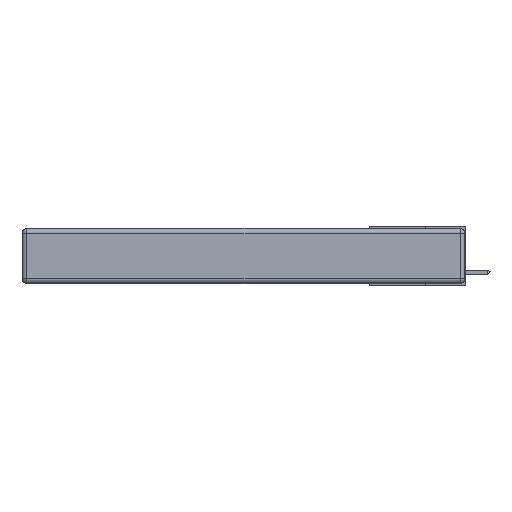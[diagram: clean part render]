
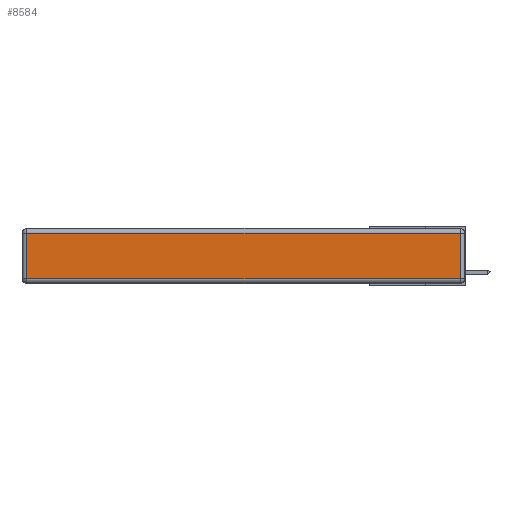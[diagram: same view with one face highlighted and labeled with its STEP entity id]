
A CAD part, left-side view. The second image highlights one B-rep face of the part: STEP entity #8584.
In plain terms, the highlighted planar face has unit normal (-1, 0, 0).
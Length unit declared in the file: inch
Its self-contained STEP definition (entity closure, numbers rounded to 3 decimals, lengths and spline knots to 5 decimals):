
#1359 = EDGE_CURVE ( 'NONE', #32406, #8533, #15320, .T. ) ;
#1415 = EDGE_CURVE ( 'NONE', #8533, #17608, #6360, .T. ) ;
#1460 = LINE ( 'NONE', #2531, #31014 ) ;
#2531 = CARTESIAN_POINT ( 'NONE',  ( 0., 2.75, -0.03 ) ) ;
#3974 = FACE_OUTER_BOUND ( 'NONE', #21183, .T. ) ;
#4182 = DIRECTION ( 'NONE',  ( 0., 0., 1. ) ) ;
#4465 = CARTESIAN_POINT ( 'NONE',  ( 0., 0.03, -0.03 ) ) ;
#6360 = LINE ( 'NONE', #19759, #19071 ) ;
#6834 = DIRECTION ( 'NONE',  ( -1., 0., 0. ) ) ;
#7842 = ORIENTED_EDGE ( 'NONE', *, *, #17301, .T. ) ;
#8352 = VECTOR ( 'NONE', #11616, 39.37008 ) ;
#8439 = ORIENTED_EDGE ( 'NONE', *, *, #1359, .T. ) ;
#8533 = VERTEX_POINT ( 'NONE', #32713 ) ;
#8584 = ADVANCED_FACE ( 'NONE', ( #3974 ), #14493, .T. ) ;
#11616 = DIRECTION ( 'NONE',  ( 0., -1., 0. ) ) ;
#12183 = LINE ( 'NONE', #15162, #33918 ) ;
#13043 = ORIENTED_EDGE ( 'NONE', *, *, #1415, .T. ) ;
#14493 = PLANE ( 'NONE',  #16801 ) ;
#15162 = CARTESIAN_POINT ( 'NONE',  ( 0., 2.72, -0.343 ) ) ;
#15320 = LINE ( 'NONE', #27313, #8352 ) ;
#16801 = AXIS2_PLACEMENT_3D ( 'NONE', #32820, #6834, #4182 ) ;
#17169 = CARTESIAN_POINT ( 'NONE',  ( 0., 2.72, -0.03 ) ) ;
#17209 = EDGE_CURVE ( 'NONE', #24010, #32406, #12183, .T. ) ;
#17301 = EDGE_CURVE ( 'NONE', #17608, #24010, #1460, .T. ) ;
#17370 = DIRECTION ( 'NONE',  ( 0., 0., 1. ) ) ;
#17608 = VERTEX_POINT ( 'NONE', #4465 ) ;
#19071 = VECTOR ( 'NONE', #17370, 39.37008 ) ;
#19759 = CARTESIAN_POINT ( 'NONE',  ( 0., 0.03, -0.343 ) ) ;
#20672 = DIRECTION ( 'NONE',  ( 0., 0., -1. ) ) ;
#21183 = EDGE_LOOP ( 'NONE', ( #8439, #13043, #7842, #26239 ) ) ;
#22844 = CARTESIAN_POINT ( 'NONE',  ( 0., 2.72, -0.313 ) ) ;
#24010 = VERTEX_POINT ( 'NONE', #17169 ) ;
#26170 = DIRECTION ( 'NONE',  ( 0., 1., 0. ) ) ;
#26239 = ORIENTED_EDGE ( 'NONE', *, *, #17209, .T. ) ;
#27313 = CARTESIAN_POINT ( 'NONE',  ( 0., 0., -0.313 ) ) ;
#31014 = VECTOR ( 'NONE', #26170, 39.37008 ) ;
#32406 = VERTEX_POINT ( 'NONE', #22844 ) ;
#32713 = CARTESIAN_POINT ( 'NONE',  ( 0., 0.03, -0.313 ) ) ;
#32820 = CARTESIAN_POINT ( 'NONE',  ( 0., 0., -0.343 ) ) ;
#33918 = VECTOR ( 'NONE', #20672, 39.37008 ) ;
